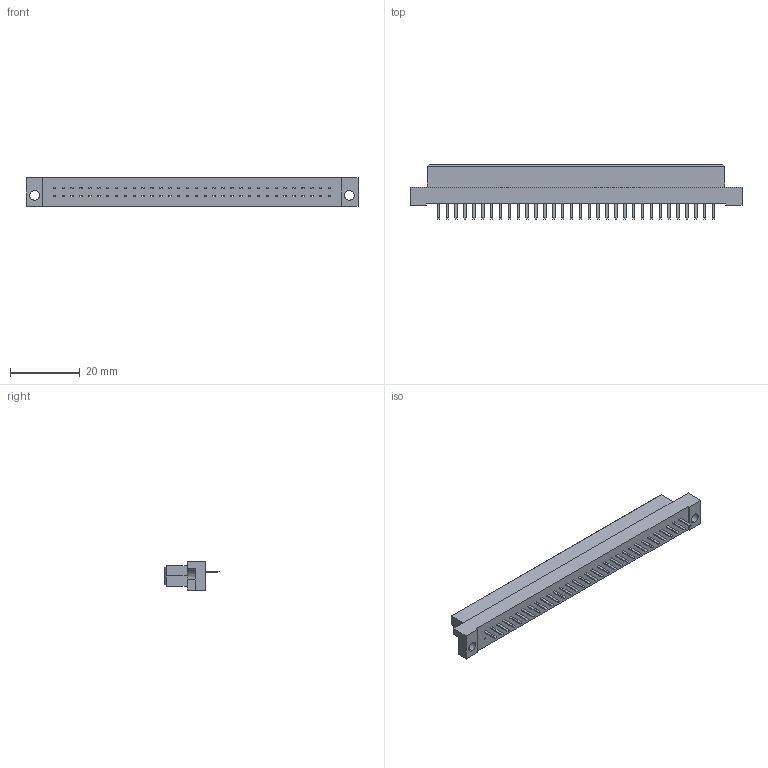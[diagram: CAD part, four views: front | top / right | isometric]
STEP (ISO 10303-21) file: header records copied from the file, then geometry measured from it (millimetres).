
FILE_DESCRIPTION (( 'STEP AP203' ), '1' );
FILE_NAME ('464-132-221-113.STEP', '2019-11-11T16:12:17', ( '' ), ( '' ), 'SwSTEP 2.0', 'SolidWorks 2020', '' );
FILE_SCHEMA (( 'CONFIG_CONTROL_DESIGN' ));
Length unit declared in the file: millimetre
Products named in the file (3): 464 Part_64; 464-132-221-113; 464-290_21
Assembly tree (33 placements, depth 2):
  464-132-221-113
    464 Part_64
    464-290_21  x32
Bounding box: 95 x 15.6 x 8.1 mm (x, y, z)
Volume: 6218.7 mm3; surface area: 6451.4 mm2
Topology: 33 solids, 33 shells, 1191 faces, 2788 edges, 1728 vertices
Faces by surface type: plane 1185, cylinder 6
Entity records: 26651 total; most frequent: CARTESIAN_POINT 4441, ORIENTED_EDGE 4336, DIRECTION 4014, EDGE_CURVE 2168, VECTOR 2156, LINE 2156, VERTEX_POINT 1356, EDGE_LOOP 1078
